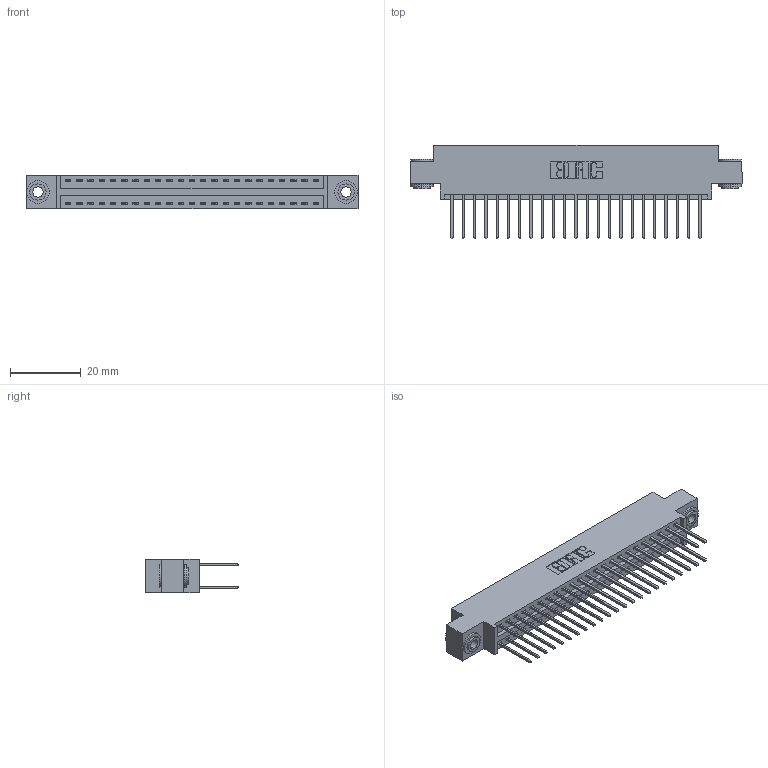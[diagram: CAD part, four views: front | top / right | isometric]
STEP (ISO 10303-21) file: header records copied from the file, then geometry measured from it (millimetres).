
FILE_DESCRIPTION (( 'STEP AP203' ), '1' );
FILE_NAME ('346-046-522-803.STEP', '2022-05-20T19:45:59', ( '' ), ( '' ), 'SwSTEP 2.0', 'SolidWorks 2020', '' );
FILE_SCHEMA (( 'CONFIG_CONTROL_DESIGN' ));
Length unit declared in the file: inch
Products named in the file (4): 345-292-001_345-293-122; 346 Part_0.170 Offset - 0.156 Dia-TH; 346-046-522-803; 345-250-002_345-250-002-102
Assembly tree (49 placements, depth 2):
  346-046-522-803
    346 Part_0.170 Offset - 0.156 Dia-TH
    345-292-001_345-293-122  x46
    345-250-002_345-250-002-102  x2
Bounding box: 93.6 x 26.42 x 9.4 mm (x, y, z)
Volume: 8944 mm3; surface area: 12970.3 mm2
Topology: 49 solids, 49 shells, 2570 faces, 7583 edges, 4990 vertices
Faces by surface type: plane 1714, cylinder 848, cone 8
Entity records: 18784 total; most frequent: CARTESIAN_POINT 3105, ORIENTED_EDGE 3030, DIRECTION 2817, EDGE_CURVE 1515, VECTOR 1267, LINE 1267, VERTEX_POINT 1006, AXIS2_PLACEMENT_3D 775
